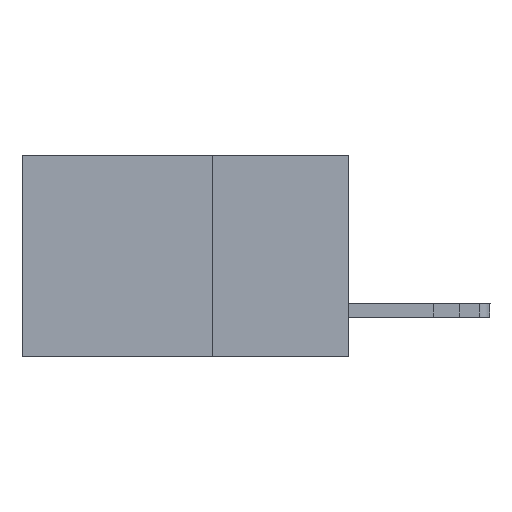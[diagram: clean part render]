
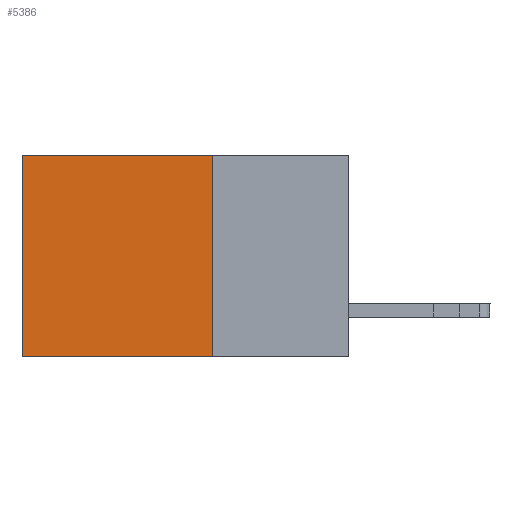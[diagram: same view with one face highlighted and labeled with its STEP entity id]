
A CAD part, left-side view. The second image highlights one B-rep face of the part: STEP entity #5386.
In plain terms, the highlighted planar face has unit normal (-1, 0, 0).
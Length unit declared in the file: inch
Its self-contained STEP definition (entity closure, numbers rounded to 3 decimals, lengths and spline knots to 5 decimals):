
#492 = ORIENTED_EDGE ( 'NONE', *, *, #18464, .T. ) ;
#1821 = VECTOR ( 'NONE', #8557, 39.37008 ) ;
#2105 = CARTESIAN_POINT ( 'NONE',  ( 0.2615, 0.6, 0. ) ) ;
#2134 = VECTOR ( 'NONE', #13072, 39.37008 ) ;
#2236 = EDGE_LOOP ( 'NONE', ( #492, #18044, #14254, #7636 ) ) ;
#3392 = DIRECTION ( 'NONE',  ( 0., 1., 0. ) ) ;
#5386 = ADVANCED_FACE ( 'NONE', ( #14949 ), #16827, .F. ) ;
#5396 = VECTOR ( 'NONE', #3392, 39.37008 ) ;
#5513 = AXIS2_PLACEMENT_3D ( 'NONE', #16848, #16789, #16785 ) ;
#6015 = CARTESIAN_POINT ( 'NONE',  ( 0.2615, 0.6, -0.37 ) ) ;
#6144 = LINE ( 'NONE', #17537, #2134 ) ;
#6416 = VERTEX_POINT ( 'NONE', #6015 ) ;
#6859 = LINE ( 'NONE', #6963, #1821 ) ;
#6963 = CARTESIAN_POINT ( 'NONE',  ( 0.2615, 0.25, -0.37 ) ) ;
#7636 = ORIENTED_EDGE ( 'NONE', *, *, #19752, .T. ) ;
#8102 = CARTESIAN_POINT ( 'NONE',  ( 0.2615, 0.25, -0.37 ) ) ;
#8352 = VECTOR ( 'NONE', #10294, 39.37008 ) ;
#8557 = DIRECTION ( 'NONE',  ( 0., 0., -1. ) ) ;
#8711 = CARTESIAN_POINT ( 'NONE',  ( 0.2615, 0.25, 0. ) ) ;
#8843 = LINE ( 'NONE', #8711, #8352 ) ;
#9637 = LINE ( 'NONE', #8102, #5396 ) ;
#9971 = VERTEX_POINT ( 'NONE', #2105 ) ;
#10294 = DIRECTION ( 'NONE',  ( 0., 1., 0. ) ) ;
#10781 = EDGE_CURVE ( 'NONE', #14555, #14699, #6859, .T. ) ;
#11773 = CARTESIAN_POINT ( 'NONE',  ( 0.2615, 0.25, 0. ) ) ;
#13072 = DIRECTION ( 'NONE',  ( 0., 0., -1. ) ) ;
#14254 = ORIENTED_EDGE ( 'NONE', *, *, #10781, .F. ) ;
#14555 = VERTEX_POINT ( 'NONE', #11773 ) ;
#14699 = VERTEX_POINT ( 'NONE', #18085 ) ;
#14949 = FACE_OUTER_BOUND ( 'NONE', #2236, .T. ) ;
#16785 = DIRECTION ( 'NONE',  ( 0., 0., -1. ) ) ;
#16789 = DIRECTION ( 'NONE',  ( 1., 0., 0. ) ) ;
#16827 = PLANE ( 'NONE',  #5513 ) ;
#16848 = CARTESIAN_POINT ( 'NONE',  ( 0.2615, 0.25, -0.37 ) ) ;
#17537 = CARTESIAN_POINT ( 'NONE',  ( 0.2615, 0.6, -0.37 ) ) ;
#18044 = ORIENTED_EDGE ( 'NONE', *, *, #18325, .F. ) ;
#18085 = CARTESIAN_POINT ( 'NONE',  ( 0.2615, 0.25, -0.37 ) ) ;
#18325 = EDGE_CURVE ( 'NONE', #14699, #6416, #9637, .T. ) ;
#18464 = EDGE_CURVE ( 'NONE', #9971, #6416, #6144, .T. ) ;
#19752 = EDGE_CURVE ( 'NONE', #14555, #9971, #8843, .T. ) ;
